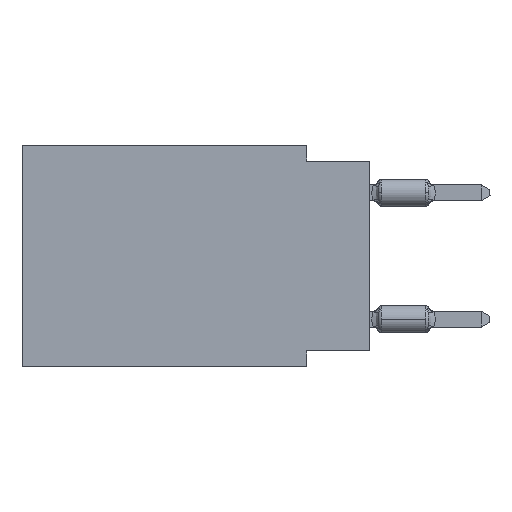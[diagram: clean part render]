
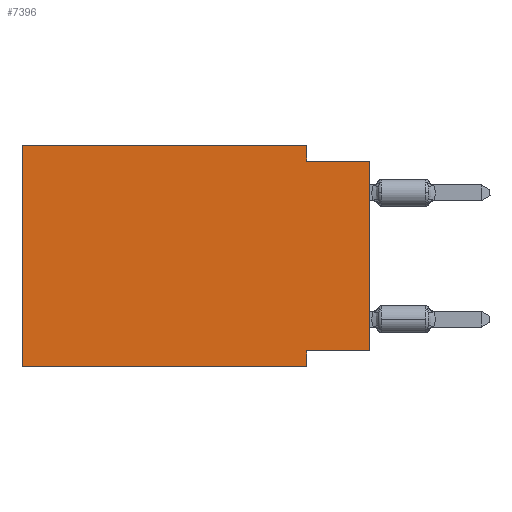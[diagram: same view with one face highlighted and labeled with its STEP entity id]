
A CAD part, left-side view. The second image highlights one B-rep face of the part: STEP entity #7396.
In plain terms, the highlighted planar face has unit normal (-1, 0, 0).
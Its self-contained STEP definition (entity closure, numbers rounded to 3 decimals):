
#1888 = ORIENTED_EDGE ( 'NONE', *, *, #50131, .F. ) ;
#2055 = EDGE_CURVE ( 'NONE', #34133, #46418, #24832, .T. ) ;
#2543 = VECTOR ( 'NONE', #24563, 1000. ) ;
#2617 = DIRECTION ( 'NONE',  ( 0., -1., 0. ) ) ;
#4017 = LINE ( 'NONE', #46194, #52968 ) ;
#4178 = CARTESIAN_POINT ( 'NONE',  ( 0., 0., 0. ) ) ;
#4505 = AXIS2_PLACEMENT_3D ( 'NONE', #29413, #28328, #45386 ) ;
#5122 = VERTEX_POINT ( 'NONE', #48595 ) ;
#6390 = CARTESIAN_POINT ( 'NONE',  ( 0., 2.54, -0.635 ) ) ;
#6965 = ORIENTED_EDGE ( 'NONE', *, *, #29997, .F. ) ;
#7396 = ADVANCED_FACE ( 'NONE', ( #20490 ), #54864, .F. ) ;
#7824 = VERTEX_POINT ( 'NONE', #18087 ) ;
#8055 = EDGE_CURVE ( 'NONE', #34632, #36373, #23109, .T. ) ;
#9240 = VERTEX_POINT ( 'NONE', #6390 ) ;
#9457 = LINE ( 'NONE', #30378, #11063 ) ;
#10668 = CARTESIAN_POINT ( 'NONE',  ( 0., 0., -8.255 ) ) ;
#11063 = VECTOR ( 'NONE', #55005, 1000. ) ;
#12458 = EDGE_CURVE ( 'NONE', #7824, #9240, #4017, .T. ) ;
#13019 = CARTESIAN_POINT ( 'NONE',  ( 0., 13.97, 0. ) ) ;
#13333 = LINE ( 'NONE', #47979, #28635 ) ;
#14611 = VERTEX_POINT ( 'NONE', #17193 ) ;
#14642 = EDGE_CURVE ( 'NONE', #14611, #36373, #52676, .T. ) ;
#15669 = VECTOR ( 'NONE', #52955, 1000. ) ;
#16973 = CARTESIAN_POINT ( 'NONE',  ( 0., 13.97, -8.89 ) ) ;
#17193 = CARTESIAN_POINT ( 'NONE',  ( 0., 2.54, -8.255 ) ) ;
#18087 = CARTESIAN_POINT ( 'NONE',  ( 0., 2.54, 0. ) ) ;
#18913 = DIRECTION ( 'NONE',  ( 0., -1., 0. ) ) ;
#20490 = FACE_OUTER_BOUND ( 'NONE', #43073, .T. ) ;
#21361 = ORIENTED_EDGE ( 'NONE', *, *, #2055, .T. ) ;
#23109 = LINE ( 'NONE', #40146, #23283 ) ;
#23283 = VECTOR ( 'NONE', #18913, 1000. ) ;
#24563 = DIRECTION ( 'NONE',  ( 0., 0., 1. ) ) ;
#24832 = LINE ( 'NONE', #4178, #2543 ) ;
#28328 = DIRECTION ( 'NONE',  ( 1., 0., 0. ) ) ;
#28635 = VECTOR ( 'NONE', #30356, 1000. ) ;
#29413 = CARTESIAN_POINT ( 'NONE',  ( 0., 13.97, 0. ) ) ;
#29997 = EDGE_CURVE ( 'NONE', #9240, #46418, #49256, .T. ) ;
#30356 = DIRECTION ( 'NONE',  ( 0., 1., 0. ) ) ;
#30378 = CARTESIAN_POINT ( 'NONE',  ( 0., 13.97, 0. ) ) ;
#30546 = VECTOR ( 'NONE', #2617, 1000. ) ;
#34133 = VERTEX_POINT ( 'NONE', #10668 ) ;
#34632 = VERTEX_POINT ( 'NONE', #16973 ) ;
#36373 = VERTEX_POINT ( 'NONE', #47555 ) ;
#36831 = ORIENTED_EDGE ( 'NONE', *, *, #8055, .T. ) ;
#38145 = DIRECTION ( 'NONE',  ( 0., 0., 1. ) ) ;
#40146 = CARTESIAN_POINT ( 'NONE',  ( 0., 13.97, -8.89 ) ) ;
#40787 = ORIENTED_EDGE ( 'NONE', *, *, #42203, .F. ) ;
#40863 = CARTESIAN_POINT ( 'NONE',  ( 0., 0., -0.635 ) ) ;
#41438 = VECTOR ( 'NONE', #38145, 1000. ) ;
#42203 = EDGE_CURVE ( 'NONE', #34133, #14611, #13333, .T. ) ;
#42263 = ORIENTED_EDGE ( 'NONE', *, *, #12458, .F. ) ;
#42879 = LINE ( 'NONE', #13019, #41438 ) ;
#43073 = EDGE_LOOP ( 'NONE', ( #21361, #6965, #42263, #1888, #44800, #36831, #49236, #40787 ) ) ;
#44800 = ORIENTED_EDGE ( 'NONE', *, *, #50547, .F. ) ;
#45386 = DIRECTION ( 'NONE',  ( 0., 0., -1. ) ) ;
#46194 = CARTESIAN_POINT ( 'NONE',  ( 0., 2.54, 0. ) ) ;
#46418 = VERTEX_POINT ( 'NONE', #52429 ) ;
#47555 = CARTESIAN_POINT ( 'NONE',  ( 0., 2.54, -8.89 ) ) ;
#47979 = CARTESIAN_POINT ( 'NONE',  ( 0., 0., -8.255 ) ) ;
#48595 = CARTESIAN_POINT ( 'NONE',  ( 0., 13.97, 0. ) ) ;
#49236 = ORIENTED_EDGE ( 'NONE', *, *, #14642, .F. ) ;
#49256 = LINE ( 'NONE', #40863, #30546 ) ;
#50131 = EDGE_CURVE ( 'NONE', #5122, #7824, #9457, .T. ) ;
#50547 = EDGE_CURVE ( 'NONE', #34632, #5122, #42879, .T. ) ;
#51948 = DIRECTION ( 'NONE',  ( 0., 0., -1. ) ) ;
#52407 = CARTESIAN_POINT ( 'NONE',  ( 0., 2.54, -8.89 ) ) ;
#52429 = CARTESIAN_POINT ( 'NONE',  ( 0., 0., -0.635 ) ) ;
#52676 = LINE ( 'NONE', #52407, #15669 ) ;
#52955 = DIRECTION ( 'NONE',  ( 0., 0., -1. ) ) ;
#52968 = VECTOR ( 'NONE', #51948, 1000. ) ;
#54864 = PLANE ( 'NONE',  #4505 ) ;
#55005 = DIRECTION ( 'NONE',  ( 0., -1., 0. ) ) ;
